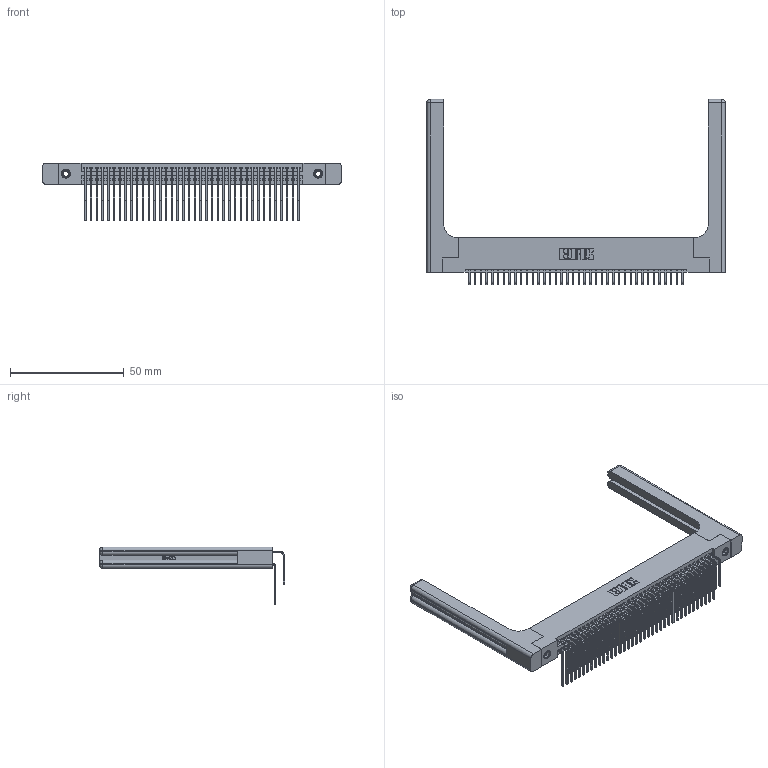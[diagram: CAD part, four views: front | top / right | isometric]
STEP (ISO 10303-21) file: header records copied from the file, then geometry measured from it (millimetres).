
FILE_DESCRIPTION (( 'STEP AP203' ), '1' );
FILE_NAME ('345-076-559-258.STEP', '2019-10-31T13:57:52', ( '' ), ( '' ), 'SwSTEP 2.0', 'SolidWorks 2016', '' );
FILE_SCHEMA (( 'CONFIG_CONTROL_DESIGN' ));
Length unit declared in the file: inch
Products named in the file (6): 345-292-001_559 Tail - 2; 345 Part_Flush Mounting Lugs - 0.156 Dia-TH; 345-292-001_558 559 Tail - 1; 345-220-058_345-220-058; 345-076-559-258; 345-250-001_345-250-001-102
Assembly tree (81 placements, depth 2):
  345-076-559-258
    345 Part_Flush Mounting Lugs - 0.156 Dia-TH
    345-292-001_558 559 Tail - 1  x38
    345-292-001_559 Tail - 2  x38
    345-250-001_345-250-001-102  x2
    345-220-058_345-220-058  x2
Bounding box: 131.55 x 81.52 x 25.53 mm (x, y, z)
Volume: 21655 mm3; surface area: 26525.1 mm2
Topology: 81 solids, 81 shells, 4334 faces, 12787 edges, 8402 vertices
Faces by surface type: plane 2888, cylinder 1386, bspline 36, cone 12, sphere 8, torus 4
Entity records: 37188 total; most frequent: CARTESIAN_POINT 7276, ORIENTED_EDGE 5956, DIRECTION 5326, EDGE_CURVE 2978, VECTOR 2562, LINE 2562, VERTEX_POINT 1974, AXIS2_PLACEMENT_3D 1382
